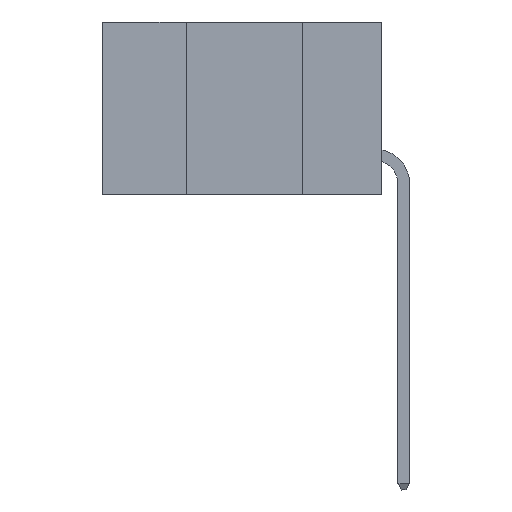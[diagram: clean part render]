
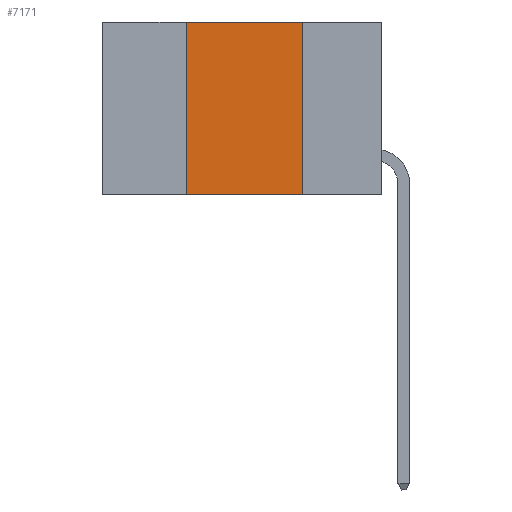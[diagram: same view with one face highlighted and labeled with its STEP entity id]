
A CAD part, left-side view. The second image highlights one B-rep face of the part: STEP entity #7171.
In plain terms, the highlighted planar face has unit normal (-1, 0, 0).
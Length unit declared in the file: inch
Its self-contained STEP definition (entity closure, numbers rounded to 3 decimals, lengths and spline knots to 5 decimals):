
#45 = DIRECTION ( 'NONE',  ( 0., -1., 0. ) ) ;
#1082 = VERTEX_POINT ( 'NONE', #13072 ) ;
#1335 = EDGE_CURVE ( 'NONE', #11723, #1082, #23408, .T. ) ;
#1792 = DIRECTION ( 'NONE',  ( 0., 0., -1. ) ) ;
#3074 = EDGE_CURVE ( 'NONE', #8502, #13088, #4473, .T. ) ;
#4473 = LINE ( 'NONE', #16624, #13881 ) ;
#5469 = PLANE ( 'NONE',  #18196 ) ;
#6328 = VECTOR ( 'NONE', #45, 39.37008 ) ;
#7146 = VECTOR ( 'NONE', #14766, 39.37008 ) ;
#7171 = ADVANCED_FACE ( 'NONE', ( #20849 ), #5469, .F. ) ;
#7574 = ORIENTED_EDGE ( 'NONE', *, *, #15181, .T. ) ;
#7755 = CARTESIAN_POINT ( 'NONE',  ( 0., 0.17, 0. ) ) ;
#8502 = VERTEX_POINT ( 'NONE', #7755 ) ;
#11723 = VERTEX_POINT ( 'NONE', #12719 ) ;
#11948 = DIRECTION ( 'NONE',  ( 0., 0., 1. ) ) ;
#12719 = CARTESIAN_POINT ( 'NONE',  ( 0., 0.42, -0.37 ) ) ;
#12972 = CARTESIAN_POINT ( 'NONE',  ( 0., 0.6, 0. ) ) ;
#13028 = DIRECTION ( 'NONE',  ( 1., 0., 0. ) ) ;
#13072 = CARTESIAN_POINT ( 'NONE',  ( 0., 0.42, 0. ) ) ;
#13088 = VERTEX_POINT ( 'NONE', #22748 ) ;
#13358 = VECTOR ( 'NONE', #11948, 39.37008 ) ;
#13724 = ORIENTED_EDGE ( 'NONE', *, *, #3074, .F. ) ;
#13881 = VECTOR ( 'NONE', #18509, 39.37008 ) ;
#14766 = DIRECTION ( 'NONE',  ( 0., -1., 0. ) ) ;
#15181 = EDGE_CURVE ( 'NONE', #11723, #13088, #16338, .T. ) ;
#15567 = ORIENTED_EDGE ( 'NONE', *, *, #1335, .F. ) ;
#16338 = LINE ( 'NONE', #22611, #6328 ) ;
#16532 = ORIENTED_EDGE ( 'NONE', *, *, #24279, .F. ) ;
#16624 = CARTESIAN_POINT ( 'NONE',  ( 0., 0.17, 0. ) ) ;
#18196 = AXIS2_PLACEMENT_3D ( 'NONE', #24308, #13028, #1792 ) ;
#18270 = EDGE_LOOP ( 'NONE', ( #13724, #16532, #15567, #7574 ) ) ;
#18509 = DIRECTION ( 'NONE',  ( 0., 0., -1. ) ) ;
#19810 = CARTESIAN_POINT ( 'NONE',  ( 0., 0.42, 0. ) ) ;
#20849 = FACE_OUTER_BOUND ( 'NONE', #18270, .T. ) ;
#21043 = LINE ( 'NONE', #12972, #7146 ) ;
#22611 = CARTESIAN_POINT ( 'NONE',  ( 0., 0.6, -0.37 ) ) ;
#22748 = CARTESIAN_POINT ( 'NONE',  ( 0., 0.17, -0.37 ) ) ;
#23408 = LINE ( 'NONE', #19810, #13358 ) ;
#24279 = EDGE_CURVE ( 'NONE', #1082, #8502, #21043, .T. ) ;
#24308 = CARTESIAN_POINT ( 'NONE',  ( 0., 0.6, 0. ) ) ;
